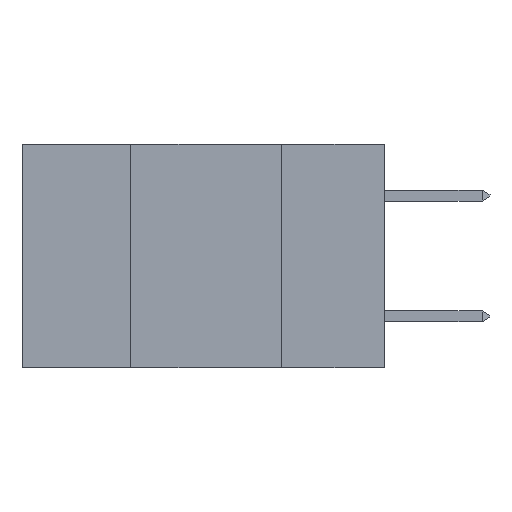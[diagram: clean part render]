
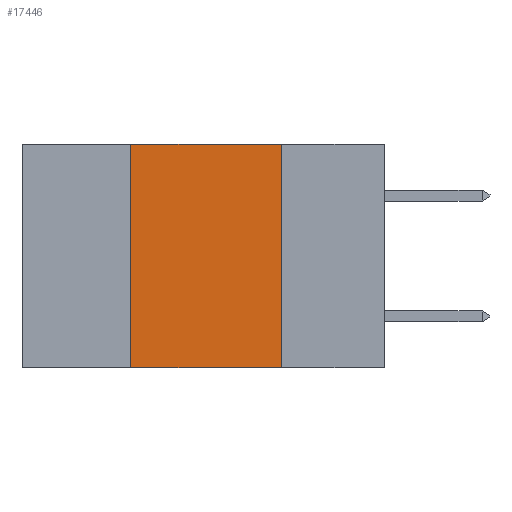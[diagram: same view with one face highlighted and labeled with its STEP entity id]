
A CAD part, left-side view. The second image highlights one B-rep face of the part: STEP entity #17446.
In plain terms, the highlighted planar face has unit normal (-1, 0, 0).
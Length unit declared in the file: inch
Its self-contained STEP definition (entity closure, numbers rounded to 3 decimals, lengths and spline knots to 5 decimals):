
#639 = VERTEX_POINT ( 'NONE', #2697 ) ;
#966 = PLANE ( 'NONE',  #11349 ) ;
#1027 = CARTESIAN_POINT ( 'NONE',  ( 0., 0.6, 0. ) ) ;
#1134 = ORIENTED_EDGE ( 'NONE', *, *, #17833, .T. ) ;
#2697 = CARTESIAN_POINT ( 'NONE',  ( 0., 0.17, 0. ) ) ;
#3385 = VECTOR ( 'NONE', #13304, 39.37008 ) ;
#3404 = FACE_OUTER_BOUND ( 'NONE', #7799, .T. ) ;
#3494 = CARTESIAN_POINT ( 'NONE',  ( 0., 0.6, -0.37 ) ) ;
#3988 = EDGE_CURVE ( 'NONE', #639, #11834, #17577, .T. ) ;
#4506 = CARTESIAN_POINT ( 'NONE',  ( 0., 0.17, -0.37 ) ) ;
#5873 = DIRECTION ( 'NONE',  ( 0., 0., 1. ) ) ;
#6603 = DIRECTION ( 'NONE',  ( 0., 0., -1. ) ) ;
#6638 = EDGE_CURVE ( 'NONE', #12678, #639, #17717, .T. ) ;
#7497 = DIRECTION ( 'NONE',  ( 0., -1., 0. ) ) ;
#7588 = CARTESIAN_POINT ( 'NONE',  ( 0., 0.17, 0. ) ) ;
#7614 = LINE ( 'NONE', #17078, #12029 ) ;
#7753 = LINE ( 'NONE', #3494, #3385 ) ;
#7799 = EDGE_LOOP ( 'NONE', ( #13600, #15777, #17859, #1134 ) ) ;
#8914 = VECTOR ( 'NONE', #7497, 39.37008 ) ;
#9399 = VERTEX_POINT ( 'NONE', #14569 ) ;
#11349 = AXIS2_PLACEMENT_3D ( 'NONE', #1027, #12187, #6603 ) ;
#11757 = CARTESIAN_POINT ( 'NONE',  ( 0., 0.6, 0. ) ) ;
#11834 = VERTEX_POINT ( 'NONE', #4506 ) ;
#12029 = VECTOR ( 'NONE', #5873, 39.37008 ) ;
#12187 = DIRECTION ( 'NONE',  ( 1., 0., 0. ) ) ;
#12310 = EDGE_CURVE ( 'NONE', #9399, #12678, #7614, .T. ) ;
#12678 = VERTEX_POINT ( 'NONE', #16349 ) ;
#13304 = DIRECTION ( 'NONE',  ( 0., -1., 0. ) ) ;
#13600 = ORIENTED_EDGE ( 'NONE', *, *, #3988, .F. ) ;
#14569 = CARTESIAN_POINT ( 'NONE',  ( 0., 0.42, -0.37 ) ) ;
#15777 = ORIENTED_EDGE ( 'NONE', *, *, #6638, .F. ) ;
#16349 = CARTESIAN_POINT ( 'NONE',  ( 0., 0.42, 0. ) ) ;
#17078 = CARTESIAN_POINT ( 'NONE',  ( 0., 0.42, 0. ) ) ;
#17423 = DIRECTION ( 'NONE',  ( 0., 0., -1. ) ) ;
#17446 = ADVANCED_FACE ( 'NONE', ( #3404 ), #966, .F. ) ;
#17577 = LINE ( 'NONE', #7588, #17778 ) ;
#17717 = LINE ( 'NONE', #11757, #8914 ) ;
#17778 = VECTOR ( 'NONE', #17423, 39.37008 ) ;
#17833 = EDGE_CURVE ( 'NONE', #9399, #11834, #7753, .T. ) ;
#17859 = ORIENTED_EDGE ( 'NONE', *, *, #12310, .F. ) ;
